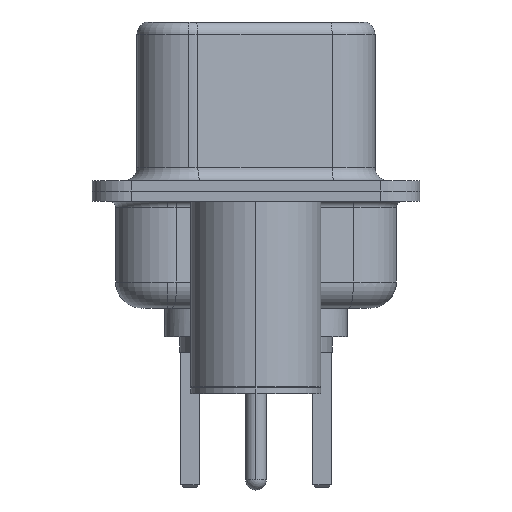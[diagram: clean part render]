
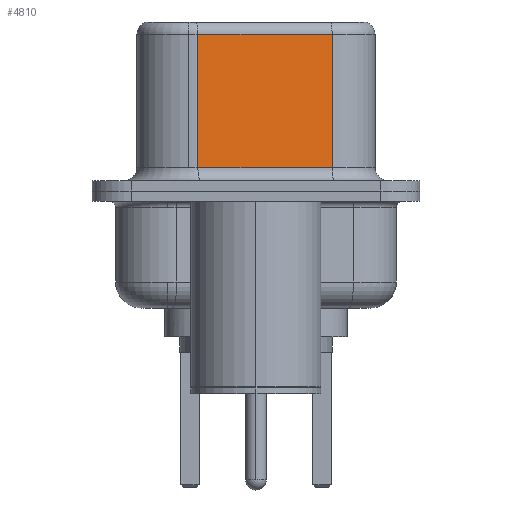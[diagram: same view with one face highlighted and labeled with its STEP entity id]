
A CAD part, left-side view. The second image highlights one B-rep face of the part: STEP entity #4810.
In plain terms, the highlighted planar face has unit normal (-0.985, -0.174, 0).
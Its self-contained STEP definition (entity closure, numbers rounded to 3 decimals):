
#274 = DIRECTION ( 'NONE',  ( 0.985, 0.174, 0. ) ) ;
#603 = VECTOR ( 'NONE', #14874, 1000. ) ;
#1607 = LINE ( 'NONE', #2258, #14870 ) ;
#1742 = DIRECTION ( 'NONE',  ( 0., 0., -1. ) ) ;
#2258 = CARTESIAN_POINT ( 'NONE',  ( 3.67, 2.233, 6.52 ) ) ;
#2808 = CARTESIAN_POINT ( 'NONE',  ( 4.58, -2.927, 0.9 ) ) ;
#3416 = CARTESIAN_POINT ( 'NONE',  ( 4.58, -2.927, 6.52 ) ) ;
#3862 = PLANE ( 'NONE',  #14103 ) ;
#4127 = ORIENTED_EDGE ( 'NONE', *, *, #21175, .T. ) ;
#4271 = CARTESIAN_POINT ( 'NONE',  ( 4.58, -2.927, 6.02 ) ) ;
#4810 = ADVANCED_FACE ( 'NONE', ( #15965 ), #3862, .F. ) ;
#5828 = DIRECTION ( 'NONE',  ( 0., 0., -1. ) ) ;
#5863 = LINE ( 'NONE', #3416, #13517 ) ;
#6753 = VERTEX_POINT ( 'NONE', #14663 ) ;
#8927 = CARTESIAN_POINT ( 'NONE',  ( 4.58, -2.927, 6.02 ) ) ;
#9105 = VERTEX_POINT ( 'NONE', #4271 ) ;
#9330 = LINE ( 'NONE', #8927, #17972 ) ;
#9708 = CARTESIAN_POINT ( 'NONE',  ( 4.58, -2.927, 6.52 ) ) ;
#10291 = EDGE_CURVE ( 'NONE', #9105, #18226, #9330, .T. ) ;
#10859 = EDGE_CURVE ( 'NONE', #21591, #6753, #13919, .T. ) ;
#12415 = DIRECTION ( 'NONE',  ( -0.174, 0.985, 0. ) ) ;
#13517 = VECTOR ( 'NONE', #1742, 1000. ) ;
#13837 = EDGE_CURVE ( 'NONE', #9105, #6753, #5863, .T. ) ;
#13919 = LINE ( 'NONE', #2808, #603 ) ;
#14103 = AXIS2_PLACEMENT_3D ( 'NONE', #9708, #274, #14603 ) ;
#14603 = DIRECTION ( 'NONE',  ( -0.174, 0.985, 0. ) ) ;
#14663 = CARTESIAN_POINT ( 'NONE',  ( 4.58, -2.927, 0.9 ) ) ;
#14812 = ORIENTED_EDGE ( 'NONE', *, *, #10291, .T. ) ;
#14870 = VECTOR ( 'NONE', #5828, 1000. ) ;
#14874 = DIRECTION ( 'NONE',  ( 0.174, -0.985, 0. ) ) ;
#15316 = CARTESIAN_POINT ( 'NONE',  ( 3.67, 2.233, 6.02 ) ) ;
#15965 = FACE_OUTER_BOUND ( 'NONE', #16350, .T. ) ;
#16350 = EDGE_LOOP ( 'NONE', ( #20875, #14812, #4127, #20722 ) ) ;
#17106 = CARTESIAN_POINT ( 'NONE',  ( 3.67, 2.233, 0.9 ) ) ;
#17972 = VECTOR ( 'NONE', #12415, 1000. ) ;
#18226 = VERTEX_POINT ( 'NONE', #15316 ) ;
#20722 = ORIENTED_EDGE ( 'NONE', *, *, #10859, .T. ) ;
#20875 = ORIENTED_EDGE ( 'NONE', *, *, #13837, .F. ) ;
#21175 = EDGE_CURVE ( 'NONE', #18226, #21591, #1607, .T. ) ;
#21591 = VERTEX_POINT ( 'NONE', #17106 ) ;
